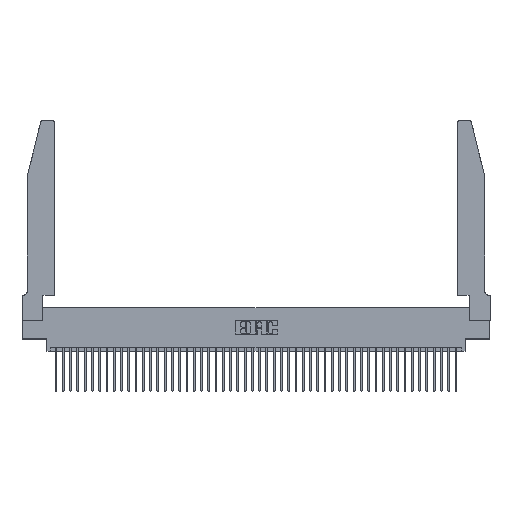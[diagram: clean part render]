
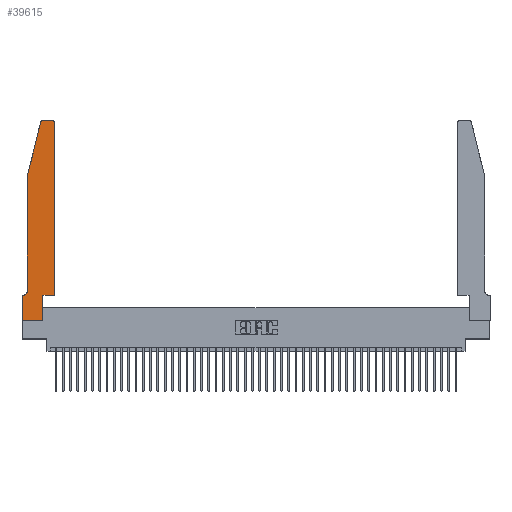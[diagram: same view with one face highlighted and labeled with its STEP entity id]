
A CAD part, top view. The second image highlights one B-rep face of the part: STEP entity #39615.
In plain terms, the highlighted planar face has unit normal (0, 0, 1).
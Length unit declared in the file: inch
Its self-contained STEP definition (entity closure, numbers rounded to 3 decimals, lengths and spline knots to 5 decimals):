
#49 = DIRECTION ( 'NONE',  ( 1., 0., 0. ) ) ;
#144 = DIRECTION ( 'NONE',  ( 1., 0., 0. ) ) ;
#337 = CARTESIAN_POINT ( 'NONE',  ( 0.0755, 2., 0.37 ) ) ;
#489 = VECTOR ( 'NONE', #21824, 39.37008 ) ;
#771 = AXIS2_PLACEMENT_3D ( 'NONE', #40830, #19163, #44422 ) ;
#1075 = ORIENTED_EDGE ( 'NONE', *, *, #33186, .T. ) ;
#1438 = CARTESIAN_POINT ( 'NONE',  ( 0.284, 2.75, 0.37 ) ) ;
#1800 = AXIS2_PLACEMENT_3D ( 'NONE', #15287, #40549, #18902 ) ;
#2352 = CARTESIAN_POINT ( 'NONE',  ( 0.0755, 0.42, 0.37 ) ) ;
#2626 = CARTESIAN_POINT ( 'NONE',  ( 0.0755, 2., 0.37 ) ) ;
#3480 = LINE ( 'NONE', #20782, #40925 ) ;
#3648 = ORIENTED_EDGE ( 'NONE', *, *, #18678, .T. ) ;
#3773 = ORIENTED_EDGE ( 'NONE', *, *, #17900, .T. ) ;
#4608 = ORIENTED_EDGE ( 'NONE', *, *, #46713, .T. ) ;
#5731 = EDGE_CURVE ( 'NONE', #29280, #6015, #17995, .T. ) ;
#6015 = VERTEX_POINT ( 'NONE', #337 ) ;
#6124 = VERTEX_POINT ( 'NONE', #11892 ) ;
#6948 = EDGE_CURVE ( 'NONE', #6124, #17327, #26839, .T. ) ;
#8440 = ORIENTED_EDGE ( 'NONE', *, *, #28673, .T. ) ;
#9675 = VERTEX_POINT ( 'NONE', #12851 ) ;
#9988 = FACE_OUTER_BOUND ( 'NONE', #34454, .T. ) ;
#10265 = CARTESIAN_POINT ( 'NONE',  ( 0., 0., 0.37 ) ) ;
#10979 = ORIENTED_EDGE ( 'NONE', *, *, #42430, .T. ) ;
#11058 = CARTESIAN_POINT ( 'NONE',  ( 0.0755, 2., 0.37 ) ) ;
#11119 = EDGE_CURVE ( 'NONE', #31400, #33966, #46314, .T. ) ;
#11461 = LINE ( 'NONE', #29258, #39169 ) ;
#11892 = CARTESIAN_POINT ( 'NONE',  ( 0.2865, 0., 0.37 ) ) ;
#12108 = DIRECTION ( 'NONE',  ( 0., 1., 0. ) ) ;
#12315 = DIRECTION ( 'NONE',  ( 0., 1., 0. ) ) ;
#12851 = CARTESIAN_POINT ( 'NONE',  ( 0.0055, 0.35, 0.37 ) ) ;
#13318 = CARTESIAN_POINT ( 'NONE',  ( 0., 0.35, 0.37 ) ) ;
#13728 = VERTEX_POINT ( 'NONE', #1438 ) ;
#15287 = CARTESIAN_POINT ( 'NONE',  ( 0.0055, 0.42, 0.37 ) ) ;
#15411 = ORIENTED_EDGE ( 'NONE', *, *, #6948, .T. ) ;
#15597 = ORIENTED_EDGE ( 'NONE', *, *, #5731, .T. ) ;
#17314 = VECTOR ( 'NONE', #12108, 39.37008 ) ;
#17327 = VERTEX_POINT ( 'NONE', #19507 ) ;
#17900 = EDGE_CURVE ( 'NONE', #13728, #29280, #46045, .T. ) ;
#17995 = LINE ( 'NONE', #2626, #19099 ) ;
#18079 = VERTEX_POINT ( 'NONE', #31610 ) ;
#18288 = CARTESIAN_POINT ( 'NONE',  ( 0., 0., 0.37 ) ) ;
#18633 = LINE ( 'NONE', #29138, #45783 ) ;
#18659 = VECTOR ( 'NONE', #12315, 39.37008 ) ;
#18678 = EDGE_CURVE ( 'NONE', #9675, #38813, #3480, .T. ) ;
#18735 = VERTEX_POINT ( 'NONE', #39332 ) ;
#18902 = DIRECTION ( 'NONE',  ( -1., 0., 0. ) ) ;
#19099 = VECTOR ( 'NONE', #24348, 39.37008 ) ;
#19163 = DIRECTION ( 'NONE',  ( 0., 0., 1. ) ) ;
#19507 = CARTESIAN_POINT ( 'NONE',  ( 0.2865, 0.35, 0.37 ) ) ;
#19862 = LINE ( 'NONE', #18288, #489 ) ;
#20028 = CARTESIAN_POINT ( 'NONE',  ( 0., 0.35, 0.37 ) ) ;
#20782 = CARTESIAN_POINT ( 'NONE',  ( 0.0755, 0.35, 0.37 ) ) ;
#21817 = DIRECTION ( 'NONE',  ( 0., 0., 1. ) ) ;
#21824 = DIRECTION ( 'NONE',  ( 0., -1., 0. ) ) ;
#23470 = PLANE ( 'NONE',  #34605 ) ;
#23608 = DIRECTION ( 'NONE',  ( 1., 0., 0. ) ) ;
#24348 = DIRECTION ( 'NONE',  ( -0.239, -0.971, 0. ) ) ;
#24579 = DIRECTION ( 'NONE',  ( 1., 0., 0. ) ) ;
#24597 = VECTOR ( 'NONE', #25365, 39.37008 ) ;
#24661 = EDGE_CURVE ( 'NONE', #33966, #18079, #24858, .T. ) ;
#24858 = CIRCLE ( 'NONE', #32193, 0.03 ) ;
#25365 = DIRECTION ( 'NONE',  ( 0., -1., 0. ) ) ;
#25753 = EDGE_CURVE ( 'NONE', #34407, #9675, #35009, .T. ) ;
#26839 = LINE ( 'NONE', #29936, #17314 ) ;
#28572 = ORIENTED_EDGE ( 'NONE', *, *, #25753, .T. ) ;
#28673 = EDGE_CURVE ( 'NONE', #17327, #31400, #11461, .T. ) ;
#29138 = CARTESIAN_POINT ( 'NONE',  ( 0.2605, 2.75, 0.37 ) ) ;
#29258 = CARTESIAN_POINT ( 'NONE',  ( 0.4505, 0.35, 0.37 ) ) ;
#29280 = VERTEX_POINT ( 'NONE', #46882 ) ;
#29532 = CARTESIAN_POINT ( 'NONE',  ( 0.4505, 0.35, 0.37 ) ) ;
#29936 = CARTESIAN_POINT ( 'NONE',  ( 0.2865, 0.35, 0.37 ) ) ;
#31400 = VERTEX_POINT ( 'NONE', #29532 ) ;
#31610 = CARTESIAN_POINT ( 'NONE',  ( 0.4205, 2.75, 0.37 ) ) ;
#31721 = DIRECTION ( 'NONE',  ( -1., 0., 0. ) ) ;
#32193 = AXIS2_PLACEMENT_3D ( 'NONE', #43526, #21817, #49 ) ;
#32292 = VECTOR ( 'NONE', #24579, 39.37008 ) ;
#32762 = DIRECTION ( 'NONE',  ( -1., 0., 0. ) ) ;
#33186 = EDGE_CURVE ( 'NONE', #6015, #34407, #43889, .T. ) ;
#33933 = CARTESIAN_POINT ( 'NONE',  ( 0.4505, 0.35, 0.37 ) ) ;
#33966 = VERTEX_POINT ( 'NONE', #43930 ) ;
#34407 = VERTEX_POINT ( 'NONE', #2352 ) ;
#34454 = EDGE_LOOP ( 'NONE', ( #10979, #3773, #15597, #1075, #28572, #3648, #4608, #36038, #15411, #8440, #39583, #37391 ) ) ;
#34605 = AXIS2_PLACEMENT_3D ( 'NONE', #20028, #45302, #23608 ) ;
#35009 = CIRCLE ( 'NONE', #1800, 0.07 ) ;
#36038 = ORIENTED_EDGE ( 'NONE', *, *, #37026, .T. ) ;
#37026 = EDGE_CURVE ( 'NONE', #18735, #6124, #40794, .T. ) ;
#37391 = ORIENTED_EDGE ( 'NONE', *, *, #24661, .T. ) ;
#38813 = VERTEX_POINT ( 'NONE', #13318 ) ;
#39169 = VECTOR ( 'NONE', #144, 39.37008 ) ;
#39332 = CARTESIAN_POINT ( 'NONE',  ( 0., 0., 0.37 ) ) ;
#39583 = ORIENTED_EDGE ( 'NONE', *, *, #11119, .T. ) ;
#39615 = ADVANCED_FACE ( 'NONE', ( #9988 ), #23470, .T. ) ;
#40549 = DIRECTION ( 'NONE',  ( 0., 0., -1. ) ) ;
#40794 = LINE ( 'NONE', #10265, #32292 ) ;
#40830 = CARTESIAN_POINT ( 'NONE',  ( 0.284, 2.72, 0.37 ) ) ;
#40925 = VECTOR ( 'NONE', #31721, 39.37008 ) ;
#42430 = EDGE_CURVE ( 'NONE', #18079, #13728, #18633, .T. ) ;
#43526 = CARTESIAN_POINT ( 'NONE',  ( 0.4205, 2.72, 0.37 ) ) ;
#43889 = LINE ( 'NONE', #11058, #24597 ) ;
#43930 = CARTESIAN_POINT ( 'NONE',  ( 0.4505, 2.72, 0.37 ) ) ;
#44422 = DIRECTION ( 'NONE',  ( 1., 0., 0. ) ) ;
#45302 = DIRECTION ( 'NONE',  ( 0., 0., 1. ) ) ;
#45783 = VECTOR ( 'NONE', #32762, 39.37008 ) ;
#46045 = CIRCLE ( 'NONE', #771, 0.03 ) ;
#46314 = LINE ( 'NONE', #33933, #18659 ) ;
#46713 = EDGE_CURVE ( 'NONE', #38813, #18735, #19862, .T. ) ;
#46882 = CARTESIAN_POINT ( 'NONE',  ( 0.25487, 2.72718, 0.37 ) ) ;
